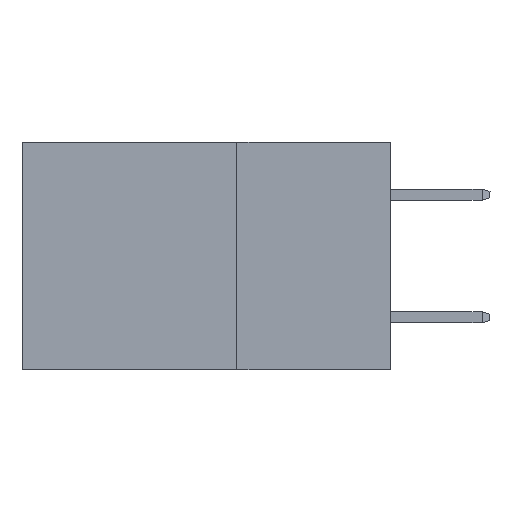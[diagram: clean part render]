
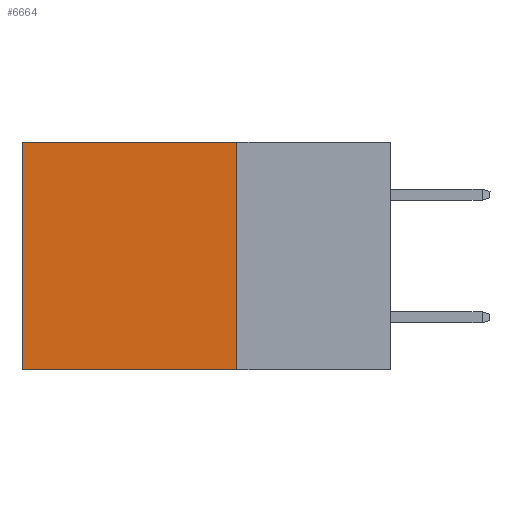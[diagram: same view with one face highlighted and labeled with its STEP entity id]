
A CAD part, left-side view. The second image highlights one B-rep face of the part: STEP entity #6664.
In plain terms, the highlighted planar face has unit normal (-1, 0, 0).
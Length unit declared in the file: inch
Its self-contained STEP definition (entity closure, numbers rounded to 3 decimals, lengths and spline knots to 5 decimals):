
#44 = CARTESIAN_POINT ( 'NONE',  ( 0.2875, 0.25, 0. ) ) ;
#201 = DIRECTION ( 'NONE',  ( 0., 1., 0. ) ) ;
#633 = ORIENTED_EDGE ( 'NONE', *, *, #6499, .T. ) ;
#681 = VERTEX_POINT ( 'NONE', #7725 ) ;
#832 = CARTESIAN_POINT ( 'NONE',  ( 0.2875, 0.25, 0. ) ) ;
#1658 = ORIENTED_EDGE ( 'NONE', *, *, #3743, .T. ) ;
#1771 = VERTEX_POINT ( 'NONE', #9851 ) ;
#2445 = DIRECTION ( 'NONE',  ( 0., 0., -1. ) ) ;
#2691 = LINE ( 'NONE', #7882, #4508 ) ;
#3168 = CARTESIAN_POINT ( 'NONE',  ( 0.2875, 0.25, 0. ) ) ;
#3385 = DIRECTION ( 'NONE',  ( 0., 0., -1. ) ) ;
#3646 = EDGE_CURVE ( 'NONE', #5844, #9940, #2691, .T. ) ;
#3743 = EDGE_CURVE ( 'NONE', #5844, #1771, #7442, .T. ) ;
#4280 = CARTESIAN_POINT ( 'NONE',  ( 0.2875, 0.25, -0.37 ) ) ;
#4508 = VECTOR ( 'NONE', #2445, 39.37008 ) ;
#4778 = DIRECTION ( 'NONE',  ( 0., 0., -1. ) ) ;
#4946 = PLANE ( 'NONE',  #9966 ) ;
#5352 = VECTOR ( 'NONE', #8730, 39.37008 ) ;
#5458 = VECTOR ( 'NONE', #4778, 39.37008 ) ;
#5844 = VERTEX_POINT ( 'NONE', #3168 ) ;
#6079 = FACE_OUTER_BOUND ( 'NONE', #6323, .T. ) ;
#6323 = EDGE_LOOP ( 'NONE', ( #633, #8295, #8633, #1658 ) ) ;
#6499 = EDGE_CURVE ( 'NONE', #1771, #681, #7553, .T. ) ;
#6664 = ADVANCED_FACE ( 'NONE', ( #6079 ), #4946, .F. ) ;
#7370 = LINE ( 'NONE', #4280, #8887 ) ;
#7442 = LINE ( 'NONE', #832, #5352 ) ;
#7553 = LINE ( 'NONE', #9360, #5458 ) ;
#7725 = CARTESIAN_POINT ( 'NONE',  ( 0.2875, 0.6, -0.37 ) ) ;
#7882 = CARTESIAN_POINT ( 'NONE',  ( 0.2875, 0.25, 0. ) ) ;
#8053 = DIRECTION ( 'NONE',  ( 1., 0., 0. ) ) ;
#8295 = ORIENTED_EDGE ( 'NONE', *, *, #9361, .F. ) ;
#8633 = ORIENTED_EDGE ( 'NONE', *, *, #3646, .F. ) ;
#8730 = DIRECTION ( 'NONE',  ( 0., 1., 0. ) ) ;
#8887 = VECTOR ( 'NONE', #201, 39.37008 ) ;
#9360 = CARTESIAN_POINT ( 'NONE',  ( 0.2875, 0.6, 0. ) ) ;
#9361 = EDGE_CURVE ( 'NONE', #9940, #681, #7370, .T. ) ;
#9548 = CARTESIAN_POINT ( 'NONE',  ( 0.2875, 0.25, -0.37 ) ) ;
#9851 = CARTESIAN_POINT ( 'NONE',  ( 0.2875, 0.6, 0. ) ) ;
#9940 = VERTEX_POINT ( 'NONE', #9548 ) ;
#9966 = AXIS2_PLACEMENT_3D ( 'NONE', #44, #8053, #3385 ) ;
